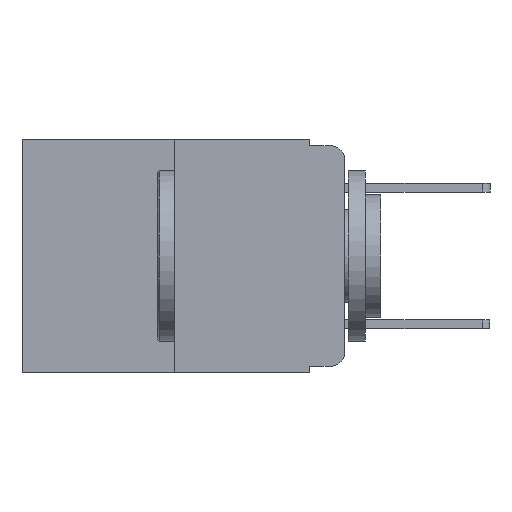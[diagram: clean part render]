
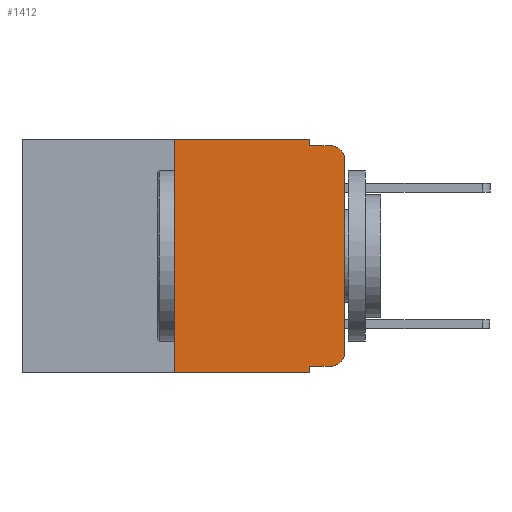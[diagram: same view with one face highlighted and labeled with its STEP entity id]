
A CAD part, left-side view. The second image highlights one B-rep face of the part: STEP entity #1412.
In plain terms, the highlighted planar face has unit normal (-1, 0, 0).
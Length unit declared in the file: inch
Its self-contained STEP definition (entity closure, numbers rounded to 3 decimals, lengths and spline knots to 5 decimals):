
#343 = CIRCLE ( 'NONE', #3316, 0.02 ) ;
#515 = CARTESIAN_POINT ( 'NONE',  ( 0., 0.051, 0. ) ) ;
#579 = ORIENTED_EDGE ( 'NONE', *, *, #5253, .T. ) ;
#663 = VERTEX_POINT ( 'NONE', #5719 ) ;
#671 = CARTESIAN_POINT ( 'NONE',  ( 0., 0.02, -0.313 ) ) ;
#772 = CARTESIAN_POINT ( 'NONE',  ( 0., 0.25, -0.343 ) ) ;
#942 = AXIS2_PLACEMENT_3D ( 'NONE', #3771, #2668, #3719 ) ;
#1242 = EDGE_CURVE ( 'NONE', #2605, #3212, #343, .T. ) ;
#1305 = VERTEX_POINT ( 'NONE', #11206 ) ;
#1412 = ADVANCED_FACE ( 'NONE', ( #8203 ), #4923, .F. ) ;
#1637 = CARTESIAN_POINT ( 'NONE',  ( 0., 0.02, -0.333 ) ) ;
#1647 = LINE ( 'NONE', #9601, #6507 ) ;
#1801 = EDGE_CURVE ( 'NONE', #663, #8758, #10021, .T. ) ;
#2016 = LINE ( 'NONE', #515, #4067 ) ;
#2353 = CARTESIAN_POINT ( 'NONE',  ( 0., 0., 0. ) ) ;
#2407 = CARTESIAN_POINT ( 'NONE',  ( 0., 0.051, -0.333 ) ) ;
#2605 = VERTEX_POINT ( 'NONE', #1637 ) ;
#2668 = DIRECTION ( 'NONE',  ( -1., 0., 0. ) ) ;
#2700 = EDGE_CURVE ( 'NONE', #4321, #11275, #2016, .T. ) ;
#2756 = CARTESIAN_POINT ( 'NONE',  ( 0., 0.051, 0. ) ) ;
#2950 = CARTESIAN_POINT ( 'NONE',  ( 0., 0.051, -0.01 ) ) ;
#3088 = ORIENTED_EDGE ( 'NONE', *, *, #1801, .T. ) ;
#3102 = ORIENTED_EDGE ( 'NONE', *, *, #4084, .F. ) ;
#3212 = VERTEX_POINT ( 'NONE', #3588 ) ;
#3316 = AXIS2_PLACEMENT_3D ( 'NONE', #671, #10823, #7214 ) ;
#3467 = DIRECTION ( 'NONE',  ( 0., -1., 0. ) ) ;
#3568 = VECTOR ( 'NONE', #10441, 39.37008 ) ;
#3588 = CARTESIAN_POINT ( 'NONE',  ( 0., 0., -0.313 ) ) ;
#3710 = EDGE_CURVE ( 'NONE', #8794, #1305, #5813, .T. ) ;
#3719 = DIRECTION ( 'NONE',  ( 0., 0., -1. ) ) ;
#3767 = VECTOR ( 'NONE', #4389, 39.37008 ) ;
#3771 = CARTESIAN_POINT ( 'NONE',  ( 0., 0.02, -0.03 ) ) ;
#3845 = DIRECTION ( 'NONE',  ( 0., 0., -1. ) ) ;
#3963 = VECTOR ( 'NONE', #11345, 39.37008 ) ;
#4027 = DIRECTION ( 'NONE',  ( 0., 0., -1. ) ) ;
#4067 = VECTOR ( 'NONE', #4027, 39.37008 ) ;
#4084 = EDGE_CURVE ( 'NONE', #11275, #8758, #5245, .T. ) ;
#4321 = VERTEX_POINT ( 'NONE', #11978 ) ;
#4389 = DIRECTION ( 'NONE',  ( 0., 0., 1. ) ) ;
#4523 = ORIENTED_EDGE ( 'NONE', *, *, #11884, .F. ) ;
#4923 = PLANE ( 'NONE',  #5035 ) ;
#4950 = CARTESIAN_POINT ( 'NONE',  ( 0., 0.051, -0.333 ) ) ;
#5035 = AXIS2_PLACEMENT_3D ( 'NONE', #12017, #10508, #3845 ) ;
#5245 = LINE ( 'NONE', #11691, #12133 ) ;
#5253 = EDGE_CURVE ( 'NONE', #8794, #7211, #1647, .T. ) ;
#5291 = CARTESIAN_POINT ( 'NONE',  ( 0., 0.051, -0.343 ) ) ;
#5719 = CARTESIAN_POINT ( 'NONE',  ( 0., 0., -0.03 ) ) ;
#5750 = VECTOR ( 'NONE', #9370, 39.37008 ) ;
#5813 = LINE ( 'NONE', #9556, #3568 ) ;
#5935 = DIRECTION ( 'NONE',  ( 0., -1., 0. ) ) ;
#5951 = DIRECTION ( 'NONE',  ( 0., -1., 0. ) ) ;
#6004 = EDGE_CURVE ( 'NONE', #1305, #4321, #7443, .T. ) ;
#6267 = LINE ( 'NONE', #2353, #3767 ) ;
#6409 = ORIENTED_EDGE ( 'NONE', *, *, #6004, .F. ) ;
#6507 = VECTOR ( 'NONE', #5951, 39.37008 ) ;
#6861 = CARTESIAN_POINT ( 'NONE',  ( 0., 0.473, 0. ) ) ;
#7207 = EDGE_CURVE ( 'NONE', #3212, #663, #6267, .T. ) ;
#7211 = VERTEX_POINT ( 'NONE', #5291 ) ;
#7214 = DIRECTION ( 'NONE',  ( 0., 0., -1. ) ) ;
#7443 = LINE ( 'NONE', #6861, #11911 ) ;
#8038 = ORIENTED_EDGE ( 'NONE', *, *, #3710, .F. ) ;
#8158 = ORIENTED_EDGE ( 'NONE', *, *, #2700, .F. ) ;
#8203 = FACE_OUTER_BOUND ( 'NONE', #10034, .T. ) ;
#8494 = LINE ( 'NONE', #2756, #5750 ) ;
#8499 = VERTEX_POINT ( 'NONE', #2407 ) ;
#8758 = VERTEX_POINT ( 'NONE', #10254 ) ;
#8794 = VERTEX_POINT ( 'NONE', #772 ) ;
#9018 = ORIENTED_EDGE ( 'NONE', *, *, #1242, .T. ) ;
#9038 = ORIENTED_EDGE ( 'NONE', *, *, #11317, .T. ) ;
#9370 = DIRECTION ( 'NONE',  ( 0., 0., -1. ) ) ;
#9556 = CARTESIAN_POINT ( 'NONE',  ( 0., 0.25, 0. ) ) ;
#9601 = CARTESIAN_POINT ( 'NONE',  ( 0., 0.473, -0.343 ) ) ;
#10021 = CIRCLE ( 'NONE', #942, 0.02 ) ;
#10034 = EDGE_LOOP ( 'NONE', ( #10517, #3088, #3102, #8158, #6409, #8038, #579, #4523, #9038, #9018 ) ) ;
#10254 = CARTESIAN_POINT ( 'NONE',  ( 0., 0.02, -0.01 ) ) ;
#10441 = DIRECTION ( 'NONE',  ( 0., 0., 1. ) ) ;
#10508 = DIRECTION ( 'NONE',  ( 1., 0., 0. ) ) ;
#10517 = ORIENTED_EDGE ( 'NONE', *, *, #7207, .T. ) ;
#10823 = DIRECTION ( 'NONE',  ( -1., 0., 0. ) ) ;
#11206 = CARTESIAN_POINT ( 'NONE',  ( 0., 0.25, 0. ) ) ;
#11275 = VERTEX_POINT ( 'NONE', #2950 ) ;
#11317 = EDGE_CURVE ( 'NONE', #8499, #2605, #11544, .T. ) ;
#11345 = DIRECTION ( 'NONE',  ( 0., -1., 0. ) ) ;
#11544 = LINE ( 'NONE', #4950, #3963 ) ;
#11691 = CARTESIAN_POINT ( 'NONE',  ( 0., 0.051, -0.01 ) ) ;
#11884 = EDGE_CURVE ( 'NONE', #8499, #7211, #8494, .T. ) ;
#11911 = VECTOR ( 'NONE', #5935, 39.37008 ) ;
#11978 = CARTESIAN_POINT ( 'NONE',  ( 0., 0.051, 0. ) ) ;
#12017 = CARTESIAN_POINT ( 'NONE',  ( 0., 0.473, 0. ) ) ;
#12133 = VECTOR ( 'NONE', #3467, 39.37008 ) ;
